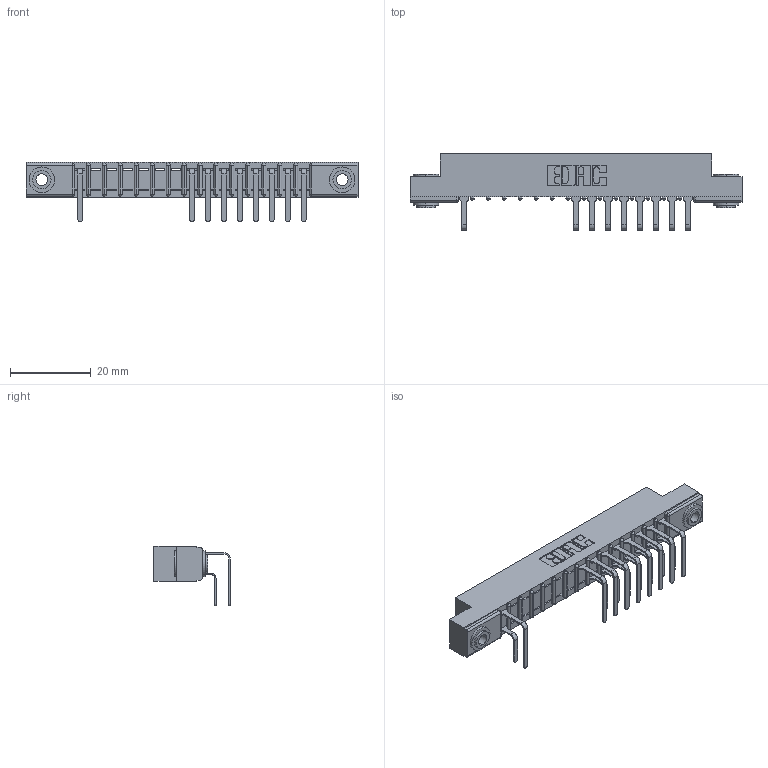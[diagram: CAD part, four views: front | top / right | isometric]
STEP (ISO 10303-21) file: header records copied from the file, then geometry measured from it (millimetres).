
FILE_DESCRIPTION (( 'STEP AP203' ), '1' );
FILE_NAME ('307-030-558-203.STEP', '2018-08-04T19:51:52', ( '' ), ( '' ), 'SwSTEP 2.0', 'SolidWorks 2016', '' );
FILE_SCHEMA (( 'CONFIG_CONTROL_DESIGN' ));
Length unit declared in the file: inch
Products named in the file (5): 307 Part_.156 Dia Mounting Holes; 307-290-001_558 559 - 1 (Single); 307-290-001_558 - 2 (Single); 345-250-002_345-250-002-102; 307-030-558-203
Assembly tree (20 placements, depth 2):
  307-030-558-203
    307 Part_.156 Dia Mounting Holes
    307-290-001_558 559 - 1 (Single)  x8
    307-290-001_558 - 2 (Single)  x9
    345-250-002_345-250-002-102  x2
Bounding box: 82.45 x 18.96 x 14.81 mm (x, y, z)
Volume: 5303.8 mm3; surface area: 8690.3 mm2
Topology: 20 solids, 20 shells, 1166 faces, 3265 edges, 2106 vertices
Faces by surface type: plane 733, cylinder 393, sphere 32, cone 8
Entity records: 18764 total; most frequent: CARTESIAN_POINT 3117, ORIENTED_EDGE 3090, DIRECTION 3065, EDGE_CURVE 1545, LINE 1165, VECTOR 1165, VERTEX_POINT 1002, AXIS2_PLACEMENT_3D 950
